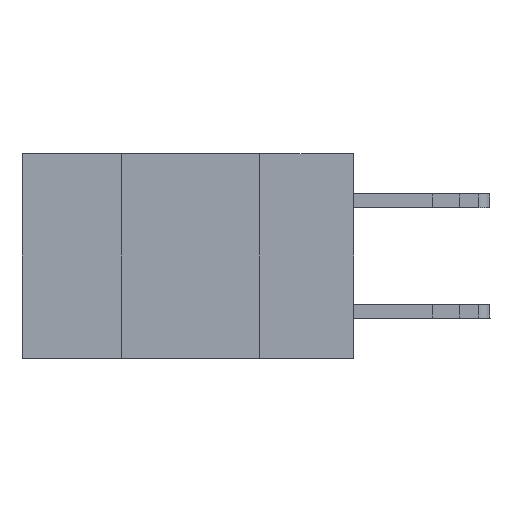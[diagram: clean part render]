
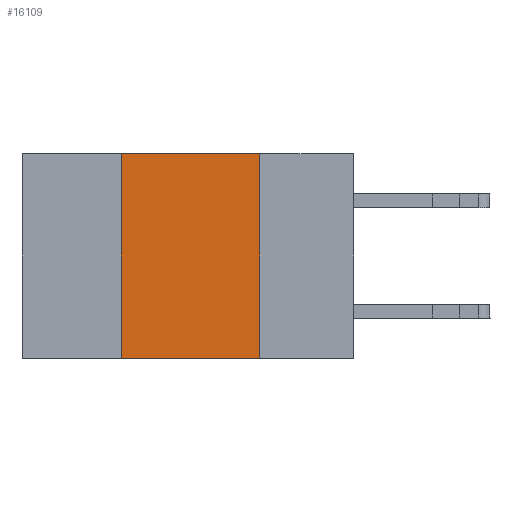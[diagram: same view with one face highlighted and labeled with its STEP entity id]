
A CAD part, left-side view. The second image highlights one B-rep face of the part: STEP entity #16109.
In plain terms, the highlighted planar face has unit normal (-1, 0, 0).
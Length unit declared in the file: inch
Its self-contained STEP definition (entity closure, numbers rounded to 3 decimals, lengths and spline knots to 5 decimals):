
#1363 = LINE ( 'NONE', #24863, #9149 ) ;
#3135 = DIRECTION ( 'NONE',  ( 0., 0., -1. ) ) ;
#3163 = DIRECTION ( 'NONE',  ( 0., -1., 0. ) ) ;
#3526 = ORIENTED_EDGE ( 'NONE', *, *, #21707, .F. ) ;
#3534 = LINE ( 'NONE', #11245, #5037 ) ;
#3784 = EDGE_LOOP ( 'NONE', ( #13349, #3526, #11517, #14231 ) ) ;
#4137 = EDGE_CURVE ( 'NONE', #9103, #10459, #23383, .T. ) ;
#4238 = AXIS2_PLACEMENT_3D ( 'NONE', #6342, #14261, #18093 ) ;
#5037 = VECTOR ( 'NONE', #3135, 39.37008 ) ;
#5433 = VECTOR ( 'NONE', #3163, 39.37008 ) ;
#5968 = CARTESIAN_POINT ( 'NONE',  ( 0., 0.17, -0.37 ) ) ;
#6342 = CARTESIAN_POINT ( 'NONE',  ( 0., 0.6, 0. ) ) ;
#6882 = LINE ( 'NONE', #16729, #5433 ) ;
#7797 = CARTESIAN_POINT ( 'NONE',  ( 0., 0.42, 0. ) ) ;
#8264 = PLANE ( 'NONE',  #4238 ) ;
#9103 = VERTEX_POINT ( 'NONE', #23943 ) ;
#9149 = VECTOR ( 'NONE', #19009, 39.37008 ) ;
#10459 = VERTEX_POINT ( 'NONE', #16825 ) ;
#11245 = CARTESIAN_POINT ( 'NONE',  ( 0., 0.17, 0. ) ) ;
#11517 = ORIENTED_EDGE ( 'NONE', *, *, #4137, .F. ) ;
#13349 = ORIENTED_EDGE ( 'NONE', *, *, #21777, .F. ) ;
#14231 = ORIENTED_EDGE ( 'NONE', *, *, #24934, .T. ) ;
#14261 = DIRECTION ( 'NONE',  ( 1., 0., 0. ) ) ;
#14735 = CARTESIAN_POINT ( 'NONE',  ( 0., 0.17, 0. ) ) ;
#15614 = DIRECTION ( 'NONE',  ( 0., 0., 1. ) ) ;
#16109 = ADVANCED_FACE ( 'NONE', ( #19989 ), #8264, .F. ) ;
#16729 = CARTESIAN_POINT ( 'NONE',  ( 0., 0.6, -0.37 ) ) ;
#16825 = CARTESIAN_POINT ( 'NONE',  ( 0., 0.42, 0. ) ) ;
#17607 = VECTOR ( 'NONE', #15614, 39.37008 ) ;
#18044 = VERTEX_POINT ( 'NONE', #14735 ) ;
#18093 = DIRECTION ( 'NONE',  ( 0., 0., -1. ) ) ;
#19009 = DIRECTION ( 'NONE',  ( 0., -1., 0. ) ) ;
#19989 = FACE_OUTER_BOUND ( 'NONE', #3784, .T. ) ;
#21707 = EDGE_CURVE ( 'NONE', #10459, #18044, #1363, .T. ) ;
#21777 = EDGE_CURVE ( 'NONE', #18044, #21840, #3534, .T. ) ;
#21840 = VERTEX_POINT ( 'NONE', #5968 ) ;
#23383 = LINE ( 'NONE', #7797, #17607 ) ;
#23943 = CARTESIAN_POINT ( 'NONE',  ( 0., 0.42, -0.37 ) ) ;
#24863 = CARTESIAN_POINT ( 'NONE',  ( 0., 0.6, 0. ) ) ;
#24934 = EDGE_CURVE ( 'NONE', #9103, #21840, #6882, .T. ) ;
